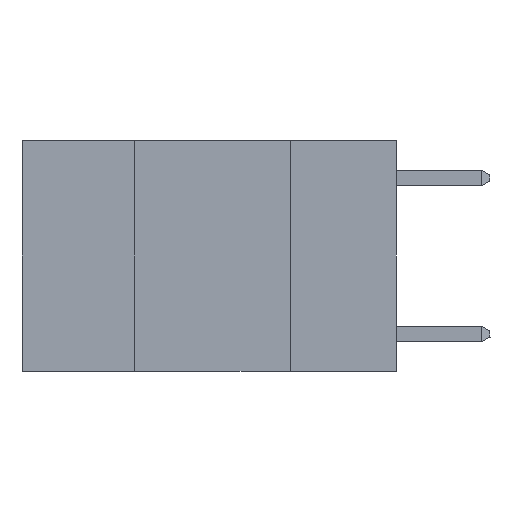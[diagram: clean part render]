
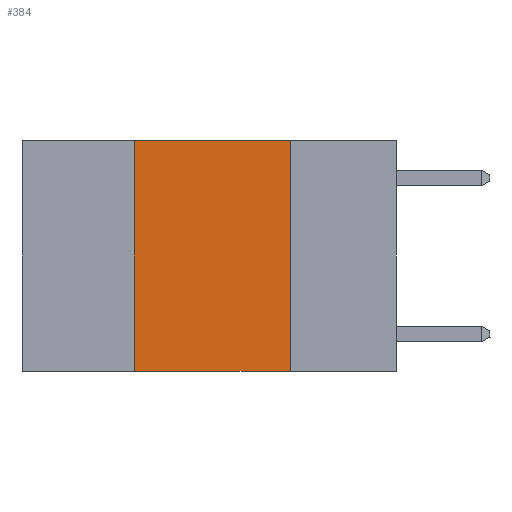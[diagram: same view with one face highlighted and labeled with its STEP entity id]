
A CAD part, left-side view. The second image highlights one B-rep face of the part: STEP entity #384.
In plain terms, the highlighted planar face has unit normal (-1, 0, 0).
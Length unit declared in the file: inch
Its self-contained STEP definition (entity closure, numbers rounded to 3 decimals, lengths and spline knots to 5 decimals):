
#383 = VERTEX_POINT ( 'NONE', #10780 ) ;
#384 = ADVANCED_FACE ( 'NONE', ( #11283 ), #3471, .F. ) ;
#477 = DIRECTION ( 'NONE',  ( 0., -1., 0. ) ) ;
#905 = DIRECTION ( 'NONE',  ( 0., -1., 0. ) ) ;
#973 = LINE ( 'NONE', #9093, #13592 ) ;
#1022 = VERTEX_POINT ( 'NONE', #9673 ) ;
#2059 = CARTESIAN_POINT ( 'NONE',  ( 0., 0.42, 0. ) ) ;
#3471 = PLANE ( 'NONE',  #4210 ) ;
#3776 = VECTOR ( 'NONE', #905, 39.37008 ) ;
#4197 = DIRECTION ( 'NONE',  ( 0., 0., -1. ) ) ;
#4210 = AXIS2_PLACEMENT_3D ( 'NONE', #8378, #11964, #4709 ) ;
#4396 = VERTEX_POINT ( 'NONE', #14343 ) ;
#4709 = DIRECTION ( 'NONE',  ( 0., 0., -1. ) ) ;
#4728 = VERTEX_POINT ( 'NONE', #11376 ) ;
#5919 = EDGE_CURVE ( 'NONE', #1022, #4396, #973, .T. ) ;
#6221 = EDGE_CURVE ( 'NONE', #383, #1022, #6686, .T. ) ;
#6686 = LINE ( 'NONE', #8398, #3776 ) ;
#7141 = EDGE_LOOP ( 'NONE', ( #12829, #10265, #8957, #15250 ) ) ;
#8378 = CARTESIAN_POINT ( 'NONE',  ( 0., 0.6, 0. ) ) ;
#8398 = CARTESIAN_POINT ( 'NONE',  ( 0., 0.6, 0. ) ) ;
#8801 = LINE ( 'NONE', #2059, #11588 ) ;
#8957 = ORIENTED_EDGE ( 'NONE', *, *, #13698, .F. ) ;
#9093 = CARTESIAN_POINT ( 'NONE',  ( 0., 0.17, 0. ) ) ;
#9162 = CARTESIAN_POINT ( 'NONE',  ( 0., 0.6, -0.37 ) ) ;
#9673 = CARTESIAN_POINT ( 'NONE',  ( 0., 0.17, 0. ) ) ;
#10265 = ORIENTED_EDGE ( 'NONE', *, *, #6221, .F. ) ;
#10780 = CARTESIAN_POINT ( 'NONE',  ( 0., 0.42, 0. ) ) ;
#11283 = FACE_OUTER_BOUND ( 'NONE', #7141, .T. ) ;
#11376 = CARTESIAN_POINT ( 'NONE',  ( 0., 0.42, -0.37 ) ) ;
#11588 = VECTOR ( 'NONE', #15412, 39.37008 ) ;
#11676 = EDGE_CURVE ( 'NONE', #4728, #4396, #15144, .T. ) ;
#11964 = DIRECTION ( 'NONE',  ( 1., 0., 0. ) ) ;
#11998 = VECTOR ( 'NONE', #477, 39.37008 ) ;
#12829 = ORIENTED_EDGE ( 'NONE', *, *, #5919, .F. ) ;
#13592 = VECTOR ( 'NONE', #4197, 39.37008 ) ;
#13698 = EDGE_CURVE ( 'NONE', #4728, #383, #8801, .T. ) ;
#14343 = CARTESIAN_POINT ( 'NONE',  ( 0., 0.17, -0.37 ) ) ;
#15144 = LINE ( 'NONE', #9162, #11998 ) ;
#15250 = ORIENTED_EDGE ( 'NONE', *, *, #11676, .T. ) ;
#15412 = DIRECTION ( 'NONE',  ( 0., 0., 1. ) ) ;
